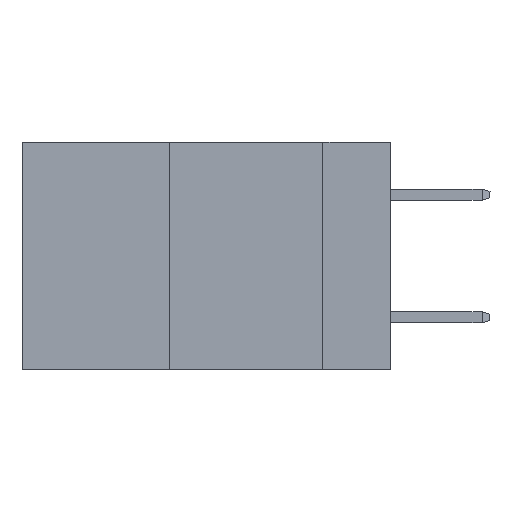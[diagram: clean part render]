
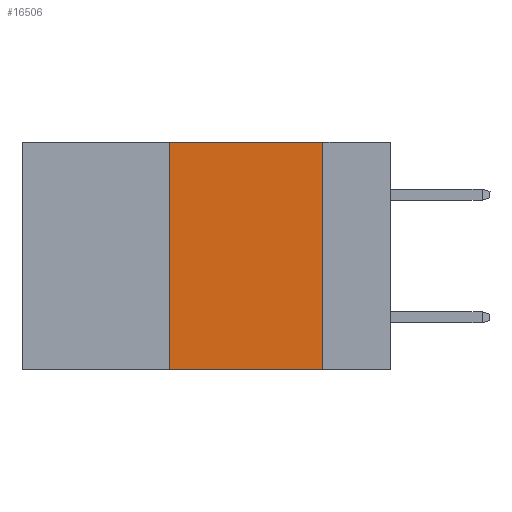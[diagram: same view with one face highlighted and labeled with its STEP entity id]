
A CAD part, left-side view. The second image highlights one B-rep face of the part: STEP entity #16506.
In plain terms, the highlighted planar face has unit normal (-1, 0, 0).
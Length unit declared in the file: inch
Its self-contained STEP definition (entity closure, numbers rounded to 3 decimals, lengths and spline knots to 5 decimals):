
#1733 = EDGE_CURVE ( 'NONE', #3467, #6984, #11404, .T. ) ;
#2308 = DIRECTION ( 'NONE',  ( 1., 0., 0. ) ) ;
#2329 = CARTESIAN_POINT ( 'NONE',  ( 0., 0.11, 0. ) ) ;
#3467 = VERTEX_POINT ( 'NONE', #5564 ) ;
#3468 = ORIENTED_EDGE ( 'NONE', *, *, #1733, .F. ) ;
#3809 = ORIENTED_EDGE ( 'NONE', *, *, #13285, .F. ) ;
#4031 = DIRECTION ( 'NONE',  ( 0., 0., -1. ) ) ;
#4974 = VECTOR ( 'NONE', #17902, 39.37008 ) ;
#5286 = CARTESIAN_POINT ( 'NONE',  ( 0., 0.11, -0.37 ) ) ;
#5564 = CARTESIAN_POINT ( 'NONE',  ( 0., 0.36, -0.37 ) ) ;
#6812 = VERTEX_POINT ( 'NONE', #18512 ) ;
#6956 = EDGE_CURVE ( 'NONE', #6812, #17721, #19831, .T. ) ;
#6984 = VERTEX_POINT ( 'NONE', #10665 ) ;
#8444 = ORIENTED_EDGE ( 'NONE', *, *, #6956, .F. ) ;
#10499 = VECTOR ( 'NONE', #4031, 39.37008 ) ;
#10665 = CARTESIAN_POINT ( 'NONE',  ( 0., 0.36, 0. ) ) ;
#11273 = FACE_OUTER_BOUND ( 'NONE', #21054, .T. ) ;
#11404 = LINE ( 'NONE', #14759, #14683 ) ;
#11644 = VECTOR ( 'NONE', #13027, 39.37008 ) ;
#12199 = CARTESIAN_POINT ( 'NONE',  ( 0., 0.6, 0. ) ) ;
#13027 = DIRECTION ( 'NONE',  ( 0., -1., 0. ) ) ;
#13194 = EDGE_CURVE ( 'NONE', #3467, #17721, #13625, .T. ) ;
#13285 = EDGE_CURVE ( 'NONE', #6984, #6812, #16544, .T. ) ;
#13625 = LINE ( 'NONE', #16171, #4974 ) ;
#13779 = DIRECTION ( 'NONE',  ( 0., 0., -1. ) ) ;
#14683 = VECTOR ( 'NONE', #18296, 39.37008 ) ;
#14759 = CARTESIAN_POINT ( 'NONE',  ( 0., 0.36, 0. ) ) ;
#16171 = CARTESIAN_POINT ( 'NONE',  ( 0., 0.6, -0.37 ) ) ;
#16506 = ADVANCED_FACE ( 'NONE', ( #11273 ), #18848, .F. ) ;
#16544 = LINE ( 'NONE', #18129, #11644 ) ;
#17193 = ORIENTED_EDGE ( 'NONE', *, *, #13194, .T. ) ;
#17721 = VERTEX_POINT ( 'NONE', #5286 ) ;
#17902 = DIRECTION ( 'NONE',  ( 0., -1., 0. ) ) ;
#18129 = CARTESIAN_POINT ( 'NONE',  ( 0., 0.6, 0. ) ) ;
#18296 = DIRECTION ( 'NONE',  ( 0., 0., 1. ) ) ;
#18512 = CARTESIAN_POINT ( 'NONE',  ( 0., 0.11, 0. ) ) ;
#18848 = PLANE ( 'NONE',  #20715 ) ;
#19831 = LINE ( 'NONE', #2329, #10499 ) ;
#20715 = AXIS2_PLACEMENT_3D ( 'NONE', #12199, #2308, #13779 ) ;
#21054 = EDGE_LOOP ( 'NONE', ( #8444, #3809, #3468, #17193 ) ) ;
